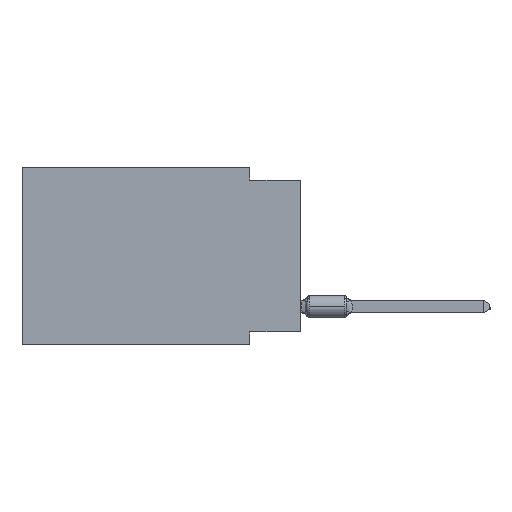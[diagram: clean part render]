
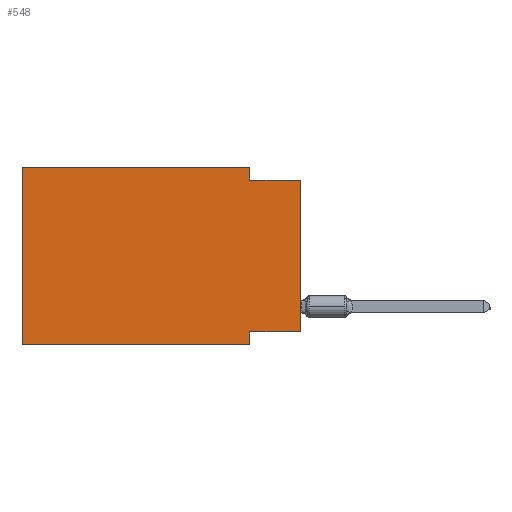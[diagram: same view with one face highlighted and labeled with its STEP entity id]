
A CAD part, left-side view. The second image highlights one B-rep face of the part: STEP entity #548.
In plain terms, the highlighted planar face has unit normal (-1, 0, 0).
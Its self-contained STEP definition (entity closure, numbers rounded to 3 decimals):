
#1 = ORIENTED_EDGE ( 'NONE', *, *, #12103, .T. ) ;
#548 = ADVANCED_FACE ( 'NONE', ( #24978 ), #20421, .F. ) ;
#820 = ORIENTED_EDGE ( 'NONE', *, *, #35841, .F. ) ;
#1830 = ORIENTED_EDGE ( 'NONE', *, *, #26180, .F. ) ;
#3251 = CARTESIAN_POINT ( 'NONE',  ( 0., 13.97, 0. ) ) ;
#3487 = CARTESIAN_POINT ( 'NONE',  ( 0., 13.97, 0. ) ) ;
#4750 = VECTOR ( 'NONE', #25205, 1000. ) ;
#5534 = CARTESIAN_POINT ( 'NONE',  ( 0., 2.54, -8.89 ) ) ;
#5870 = EDGE_CURVE ( 'NONE', #45063, #36545, #24739, .T. ) ;
#7031 = DIRECTION ( 'NONE',  ( 0., -1., 0. ) ) ;
#7493 = VERTEX_POINT ( 'NONE', #28846 ) ;
#8333 = LINE ( 'NONE', #17198, #43455 ) ;
#9821 = LINE ( 'NONE', #5534, #50432 ) ;
#12103 = EDGE_CURVE ( 'NONE', #46042, #7493, #8333, .T. ) ;
#12317 = CARTESIAN_POINT ( 'NONE',  ( 0., 13.97, 0. ) ) ;
#12957 = CARTESIAN_POINT ( 'NONE',  ( 0., 2.54, 0. ) ) ;
#13141 = LINE ( 'NONE', #48990, #44382 ) ;
#13284 = VECTOR ( 'NONE', #36627, 1000. ) ;
#13576 = ORIENTED_EDGE ( 'NONE', *, *, #32295, .F. ) ;
#14269 = CARTESIAN_POINT ( 'NONE',  ( 0., 13.97, -8.89 ) ) ;
#14498 = VECTOR ( 'NONE', #44966, 1000. ) ;
#15207 = ORIENTED_EDGE ( 'NONE', *, *, #21468, .F. ) ;
#15766 = CARTESIAN_POINT ( 'NONE',  ( 0., 13.97, -8.89 ) ) ;
#16856 = CARTESIAN_POINT ( 'NONE',  ( 0., 2.54, -8.255 ) ) ;
#17198 = CARTESIAN_POINT ( 'NONE',  ( 0., 0., 0. ) ) ;
#19112 = LINE ( 'NONE', #36048, #13284 ) ;
#20023 = CARTESIAN_POINT ( 'NONE',  ( 0., 2.54, -0.635 ) ) ;
#20421 = PLANE ( 'NONE',  #38936 ) ;
#20911 = LINE ( 'NONE', #12317, #4750 ) ;
#21424 = DIRECTION ( 'NONE',  ( 0., -1., 0. ) ) ;
#21468 = EDGE_CURVE ( 'NONE', #36545, #22120, #13141, .T. ) ;
#22120 = VERTEX_POINT ( 'NONE', #20023 ) ;
#24290 = CARTESIAN_POINT ( 'NONE',  ( 0., 0., -8.255 ) ) ;
#24386 = DIRECTION ( 'NONE',  ( 0., 0., -1. ) ) ;
#24739 = LINE ( 'NONE', #3251, #32730 ) ;
#24978 = FACE_OUTER_BOUND ( 'NONE', #27650, .T. ) ;
#25205 = DIRECTION ( 'NONE',  ( 0., 0., 1. ) ) ;
#26180 = EDGE_CURVE ( 'NONE', #22120, #7493, #52705, .T. ) ;
#27185 = DIRECTION ( 'NONE',  ( 0., 0., -1. ) ) ;
#27650 = EDGE_LOOP ( 'NONE', ( #1, #1830, #15207, #44864, #820, #42120, #13576, #56203 ) ) ;
#28774 = DIRECTION ( 'NONE',  ( 0., 0., 1. ) ) ;
#28846 = CARTESIAN_POINT ( 'NONE',  ( 0., 0., -0.635 ) ) ;
#29363 = EDGE_CURVE ( 'NONE', #53897, #49390, #48991, .T. ) ;
#32295 = EDGE_CURVE ( 'NONE', #49731, #49390, #9821, .T. ) ;
#32730 = VECTOR ( 'NONE', #7031, 1000. ) ;
#35841 = EDGE_CURVE ( 'NONE', #53897, #45063, #20911, .T. ) ;
#36048 = CARTESIAN_POINT ( 'NONE',  ( 0., 0., -8.255 ) ) ;
#36545 = VERTEX_POINT ( 'NONE', #12957 ) ;
#36627 = DIRECTION ( 'NONE',  ( 0., 1., 0. ) ) ;
#38936 = AXIS2_PLACEMENT_3D ( 'NONE', #3487, #41971, #51400 ) ;
#41771 = VECTOR ( 'NONE', #21424, 1000. ) ;
#41971 = DIRECTION ( 'NONE',  ( 1., 0., 0. ) ) ;
#42120 = ORIENTED_EDGE ( 'NONE', *, *, #29363, .T. ) ;
#43455 = VECTOR ( 'NONE', #28774, 1000. ) ;
#44382 = VECTOR ( 'NONE', #27185, 1000. ) ;
#44864 = ORIENTED_EDGE ( 'NONE', *, *, #5870, .F. ) ;
#44966 = DIRECTION ( 'NONE',  ( 0., -1., 0. ) ) ;
#45063 = VERTEX_POINT ( 'NONE', #49158 ) ;
#46042 = VERTEX_POINT ( 'NONE', #24290 ) ;
#46218 = EDGE_CURVE ( 'NONE', #46042, #49731, #19112, .T. ) ;
#47539 = CARTESIAN_POINT ( 'NONE',  ( 0., 0., -0.635 ) ) ;
#48990 = CARTESIAN_POINT ( 'NONE',  ( 0., 2.54, 0. ) ) ;
#48991 = LINE ( 'NONE', #14269, #14498 ) ;
#49158 = CARTESIAN_POINT ( 'NONE',  ( 0., 13.97, 0. ) ) ;
#49390 = VERTEX_POINT ( 'NONE', #53939 ) ;
#49731 = VERTEX_POINT ( 'NONE', #16856 ) ;
#50432 = VECTOR ( 'NONE', #24386, 1000. ) ;
#51400 = DIRECTION ( 'NONE',  ( 0., 0., -1. ) ) ;
#52705 = LINE ( 'NONE', #47539, #41771 ) ;
#53897 = VERTEX_POINT ( 'NONE', #15766 ) ;
#53939 = CARTESIAN_POINT ( 'NONE',  ( 0., 2.54, -8.89 ) ) ;
#56203 = ORIENTED_EDGE ( 'NONE', *, *, #46218, .F. ) ;
